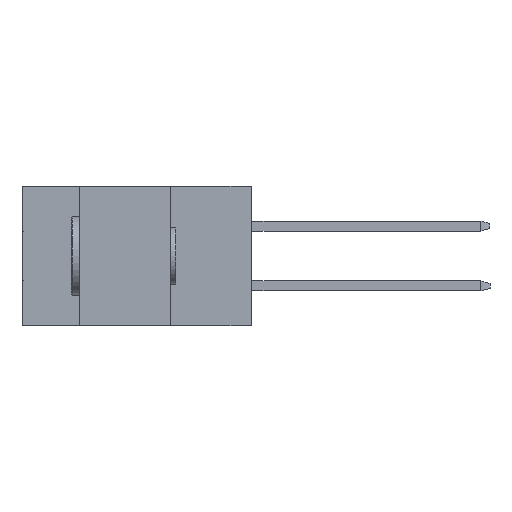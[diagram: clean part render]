
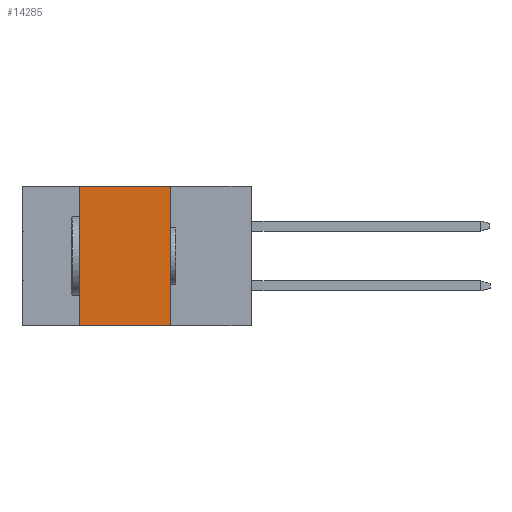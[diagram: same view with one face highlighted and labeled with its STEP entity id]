
A CAD part, left-side view. The second image highlights one B-rep face of the part: STEP entity #14285.
In plain terms, the highlighted planar face has unit normal (-1, 0, 0).
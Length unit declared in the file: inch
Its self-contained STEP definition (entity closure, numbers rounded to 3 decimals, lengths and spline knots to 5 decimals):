
#107 = EDGE_CURVE ( 'NONE', #6468, #20557, #20093, .T. ) ;
#866 = CARTESIAN_POINT ( 'NONE',  ( 0., 0.254, 0. ) ) ;
#1675 = DIRECTION ( 'NONE',  ( 1., 0., 0. ) ) ;
#1874 = CARTESIAN_POINT ( 'NONE',  ( 0., 0.254, -0.437 ) ) ;
#2018 = VECTOR ( 'NONE', #9106, 39.37008 ) ;
#2718 = AXIS2_PLACEMENT_3D ( 'NONE', #20126, #1675, #6998 ) ;
#2732 = LINE ( 'NONE', #13254, #15907 ) ;
#3735 = VECTOR ( 'NONE', #20421, 39.37008 ) ;
#3894 = CARTESIAN_POINT ( 'NONE',  ( 0., 0.54, -0.437 ) ) ;
#4321 = DIRECTION ( 'NONE',  ( 0., -1., 0. ) ) ;
#4548 = LINE ( 'NONE', #18655, #19022 ) ;
#6010 = EDGE_CURVE ( 'NONE', #19530, #9968, #2732, .T. ) ;
#6468 = VERTEX_POINT ( 'NONE', #866 ) ;
#6998 = DIRECTION ( 'NONE',  ( 0., 0., -1. ) ) ;
#8856 = ORIENTED_EDGE ( 'NONE', *, *, #6010, .F. ) ;
#9106 = DIRECTION ( 'NONE',  ( 0., 0., -1. ) ) ;
#9968 = VERTEX_POINT ( 'NONE', #14036 ) ;
#10883 = EDGE_CURVE ( 'NONE', #9968, #6468, #22199, .T. ) ;
#11964 = CARTESIAN_POINT ( 'NONE',  ( 0., 0.254, -0.437 ) ) ;
#13067 = CARTESIAN_POINT ( 'NONE',  ( 0., 0.72, 0. ) ) ;
#13254 = CARTESIAN_POINT ( 'NONE',  ( 0., 0.54, -0.437 ) ) ;
#14036 = CARTESIAN_POINT ( 'NONE',  ( 0., 0.54, 0. ) ) ;
#14285 = ADVANCED_FACE ( 'NONE', ( #15994 ), #23224, .F. ) ;
#15907 = VECTOR ( 'NONE', #16572, 39.37008 ) ;
#15994 = FACE_OUTER_BOUND ( 'NONE', #16580, .T. ) ;
#16572 = DIRECTION ( 'NONE',  ( 0., 0., 1. ) ) ;
#16580 = EDGE_LOOP ( 'NONE', ( #20618, #22909, #8856, #16720 ) ) ;
#16720 = ORIENTED_EDGE ( 'NONE', *, *, #21955, .T. ) ;
#18655 = CARTESIAN_POINT ( 'NONE',  ( 0., 0.72, -0.437 ) ) ;
#19022 = VECTOR ( 'NONE', #4321, 39.37008 ) ;
#19530 = VERTEX_POINT ( 'NONE', #3894 ) ;
#20093 = LINE ( 'NONE', #1874, #2018 ) ;
#20126 = CARTESIAN_POINT ( 'NONE',  ( 0., 0.72, 0. ) ) ;
#20421 = DIRECTION ( 'NONE',  ( 0., -1., 0. ) ) ;
#20557 = VERTEX_POINT ( 'NONE', #11964 ) ;
#20618 = ORIENTED_EDGE ( 'NONE', *, *, #107, .F. ) ;
#21955 = EDGE_CURVE ( 'NONE', #19530, #20557, #4548, .T. ) ;
#22199 = LINE ( 'NONE', #13067, #3735 ) ;
#22909 = ORIENTED_EDGE ( 'NONE', *, *, #10883, .F. ) ;
#23224 = PLANE ( 'NONE',  #2718 ) ;
